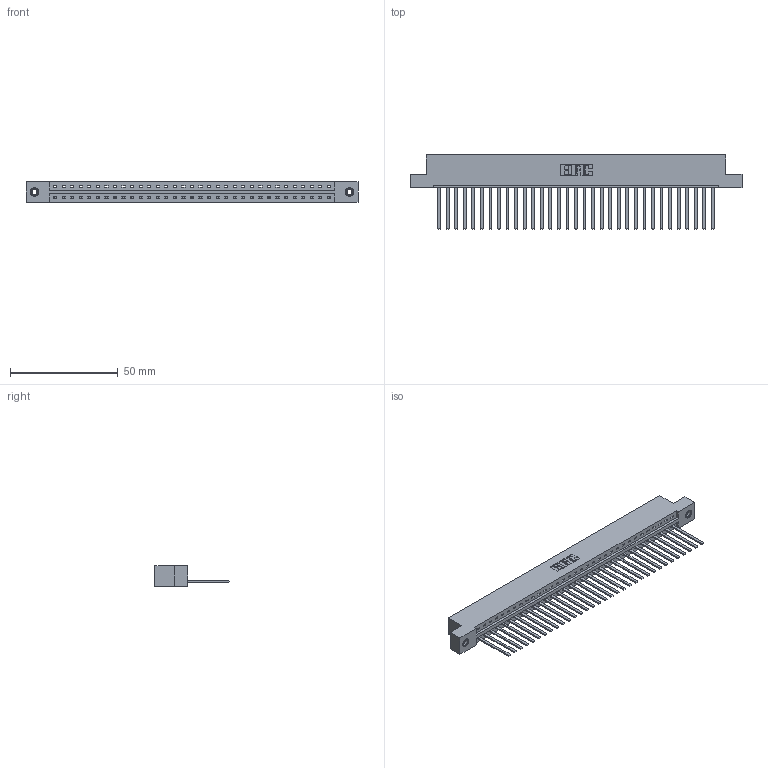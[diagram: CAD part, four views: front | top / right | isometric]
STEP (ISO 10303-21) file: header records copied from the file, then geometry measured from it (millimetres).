
FILE_DESCRIPTION (( 'STEP AP203' ), '1' );
FILE_NAME ('387-033-544-108.STEP', '2019-10-03T22:32:19', ( '' ), ( '' ), 'SwSTEP 2.0', 'SolidWorks 2016', '' );
FILE_SCHEMA (( 'CONFIG_CONTROL_DESIGN' ));
Length unit declared in the file: inch
Products named in the file (4): 345-292-001_345-293-144; 387-033-544-108; 345-250-001_345-250-003-102; 337 Part_Flush Mounting Lugs - 0.156 Dia-TI
Assembly tree (36 placements, depth 2):
  387-033-544-108
    337 Part_Flush Mounting Lugs - 0.156 Dia-TI
    345-292-001_345-293-144  x33
    345-250-001_345-250-003-102  x2
Bounding box: 153.77 x 34.3 x 9.4 mm (x, y, z)
Volume: 16245 mm3; surface area: 18023.8 mm2
Topology: 36 solids, 36 shells, 2022 faces, 6057 edges, 3986 vertices
Faces by surface type: plane 1488, cylinder 518, cone 12, torus 4
Entity records: 26696 total; most frequent: CARTESIAN_POINT 4628, ORIENTED_EDGE 4590, DIRECTION 3943, EDGE_CURVE 2295, VECTOR 2151, LINE 2151, VERTEX_POINT 1524, AXIS2_PLACEMENT_3D 896
